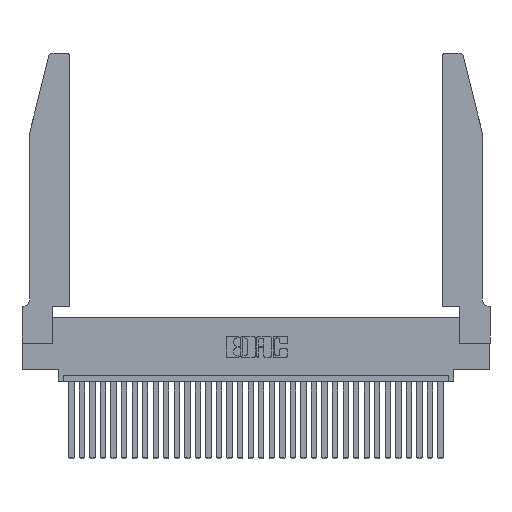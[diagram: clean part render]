
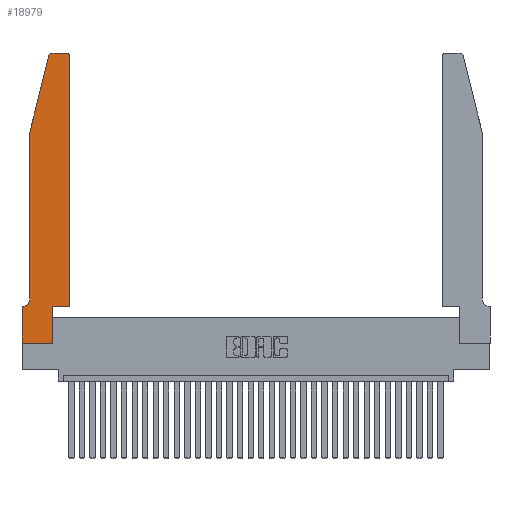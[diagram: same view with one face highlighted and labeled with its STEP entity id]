
A CAD part, top view. The second image highlights one B-rep face of the part: STEP entity #18979.
In plain terms, the highlighted planar face has unit normal (0, 0, 1).
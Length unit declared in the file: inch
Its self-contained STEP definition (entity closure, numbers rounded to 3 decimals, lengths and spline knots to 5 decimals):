
#83 = LINE ( 'NONE', #4993, #12623 ) ;
#349 = DIRECTION ( 'NONE',  ( 0., 1., 0. ) ) ;
#576 = DIRECTION ( 'NONE',  ( -1., 0., 0. ) ) ;
#654 = ORIENTED_EDGE ( 'NONE', *, *, #13467, .T. ) ;
#873 = PLANE ( 'NONE',  #4785 ) ;
#949 = ORIENTED_EDGE ( 'NONE', *, *, #26292, .T. ) ;
#970 = CARTESIAN_POINT ( 'NONE',  ( 0.2865, 0., 0.37 ) ) ;
#1658 = VECTOR ( 'NONE', #25198, 39.37008 ) ;
#1722 = VECTOR ( 'NONE', #32138, 39.37008 ) ;
#1872 = ORIENTED_EDGE ( 'NONE', *, *, #31669, .T. ) ;
#2252 = VERTEX_POINT ( 'NONE', #970 ) ;
#2437 = CARTESIAN_POINT ( 'NONE',  ( 0.2605, 2.75, 0.37 ) ) ;
#2609 = EDGE_CURVE ( 'NONE', #12792, #5001, #16962, .T. ) ;
#2851 = CARTESIAN_POINT ( 'NONE',  ( 0.4505, 0.35, 0.37 ) ) ;
#3539 = CARTESIAN_POINT ( 'NONE',  ( 0.0755, 0.42, 0.37 ) ) ;
#4785 = AXIS2_PLACEMENT_3D ( 'NONE', #5818, #31014, #18447 ) ;
#4786 = VERTEX_POINT ( 'NONE', #20227 ) ;
#4993 = CARTESIAN_POINT ( 'NONE',  ( 0.4505, 0.35, 0.37 ) ) ;
#5001 = VERTEX_POINT ( 'NONE', #8666 ) ;
#5353 = VERTEX_POINT ( 'NONE', #7013 ) ;
#5653 = CIRCLE ( 'NONE', #23288, 0.03 ) ;
#5818 = CARTESIAN_POINT ( 'NONE',  ( 0., 0.35, 0.37 ) ) ;
#6017 = DIRECTION ( 'NONE',  ( 1., 0., 0. ) ) ;
#6213 = VECTOR ( 'NONE', #12584, 39.37008 ) ;
#6500 = CARTESIAN_POINT ( 'NONE',  ( 0.25487, 2.72718, 0.37 ) ) ;
#6783 = CARTESIAN_POINT ( 'NONE',  ( 0.0755, 0.35, 0.37 ) ) ;
#7013 = CARTESIAN_POINT ( 'NONE',  ( 0., 0.35, 0.37 ) ) ;
#7657 = LINE ( 'NONE', #15133, #13528 ) ;
#7698 = EDGE_CURVE ( 'NONE', #23932, #23262, #24524, .T. ) ;
#7699 = ORIENTED_EDGE ( 'NONE', *, *, #22685, .T. ) ;
#7839 = CARTESIAN_POINT ( 'NONE',  ( 0.0055, 0.35, 0.37 ) ) ;
#7915 = CARTESIAN_POINT ( 'NONE',  ( 0.0055, 0.42, 0.37 ) ) ;
#8496 = EDGE_CURVE ( 'NONE', #15314, #18345, #83, .T. ) ;
#8666 = CARTESIAN_POINT ( 'NONE',  ( 0.284, 2.75, 0.37 ) ) ;
#9888 = AXIS2_PLACEMENT_3D ( 'NONE', #7915, #30484, #576 ) ;
#9970 = LINE ( 'NONE', #24410, #16223 ) ;
#10992 = CARTESIAN_POINT ( 'NONE',  ( 0.0755, 2., 0.37 ) ) ;
#11444 = LINE ( 'NONE', #6783, #19309 ) ;
#11681 = ORIENTED_EDGE ( 'NONE', *, *, #8496, .T. ) ;
#11913 = AXIS2_PLACEMENT_3D ( 'NONE', #13554, #18541, #6017 ) ;
#12584 = DIRECTION ( 'NONE',  ( 0., 1., 0. ) ) ;
#12623 = VECTOR ( 'NONE', #27321, 39.37008 ) ;
#12693 = EDGE_CURVE ( 'NONE', #5001, #23932, #5653, .T. ) ;
#12792 = VERTEX_POINT ( 'NONE', #27044 ) ;
#12850 = EDGE_CURVE ( 'NONE', #4786, #2252, #25303, .T. ) ;
#13062 = EDGE_LOOP ( 'NONE', ( #16958, #14139, #15153, #7699, #27635, #29638, #1872, #18734, #949, #11681, #30014, #654 ) ) ;
#13467 = EDGE_CURVE ( 'NONE', #32119, #12792, #19320, .T. ) ;
#13528 = VECTOR ( 'NONE', #349, 39.37008 ) ;
#13554 = CARTESIAN_POINT ( 'NONE',  ( 0.4205, 2.72, 0.37 ) ) ;
#14139 = ORIENTED_EDGE ( 'NONE', *, *, #12693, .T. ) ;
#14757 = CARTESIAN_POINT ( 'NONE',  ( 0.0755, 2., 0.37 ) ) ;
#15133 = CARTESIAN_POINT ( 'NONE',  ( 0.2865, 0.35, 0.37 ) ) ;
#15153 = ORIENTED_EDGE ( 'NONE', *, *, #7698, .T. ) ;
#15314 = VERTEX_POINT ( 'NONE', #26490 ) ;
#15515 = DIRECTION ( 'NONE',  ( -1., 0., 0. ) ) ;
#16223 = VECTOR ( 'NONE', #16707, 39.37008 ) ;
#16453 = VERTEX_POINT ( 'NONE', #3539 ) ;
#16707 = DIRECTION ( 'NONE',  ( 0., -1., 0. ) ) ;
#16958 = ORIENTED_EDGE ( 'NONE', *, *, #2609, .T. ) ;
#16962 = LINE ( 'NONE', #2437, #1658 ) ;
#17062 = EDGE_CURVE ( 'NONE', #28732, #5353, #11444, .T. ) ;
#17802 = VECTOR ( 'NONE', #25663, 39.37008 ) ;
#18345 = VERTEX_POINT ( 'NONE', #2851 ) ;
#18447 = DIRECTION ( 'NONE',  ( 1., 0., 0. ) ) ;
#18541 = DIRECTION ( 'NONE',  ( 0., 0., 1. ) ) ;
#18734 = ORIENTED_EDGE ( 'NONE', *, *, #12850, .T. ) ;
#18979 = ADVANCED_FACE ( 'NONE', ( #26708 ), #873, .T. ) ;
#19309 = VECTOR ( 'NONE', #15515, 39.37008 ) ;
#19320 = CIRCLE ( 'NONE', #11913, 0.03 ) ;
#20129 = EDGE_CURVE ( 'NONE', #18345, #32119, #28972, .T. ) ;
#20227 = CARTESIAN_POINT ( 'NONE',  ( 0., 0., 0.37 ) ) ;
#20309 = CARTESIAN_POINT ( 'NONE',  ( 0.4505, 0.35, 0.37 ) ) ;
#20522 = LINE ( 'NONE', #14757, #24057 ) ;
#21800 = CARTESIAN_POINT ( 'NONE',  ( 0.0755, 2., 0.37 ) ) ;
#22073 = CARTESIAN_POINT ( 'NONE',  ( 0., 0., 0.37 ) ) ;
#22685 = EDGE_CURVE ( 'NONE', #23262, #16453, #20522, .T. ) ;
#23262 = VERTEX_POINT ( 'NONE', #21800 ) ;
#23288 = AXIS2_PLACEMENT_3D ( 'NONE', #28017, #30804, #30583 ) ;
#23932 = VERTEX_POINT ( 'NONE', #6500 ) ;
#24057 = VECTOR ( 'NONE', #27346, 39.37008 ) ;
#24410 = CARTESIAN_POINT ( 'NONE',  ( 0., 0., 0.37 ) ) ;
#24524 = LINE ( 'NONE', #10992, #17802 ) ;
#25198 = DIRECTION ( 'NONE',  ( -1., 0., 0. ) ) ;
#25303 = LINE ( 'NONE', #22073, #1722 ) ;
#25390 = CARTESIAN_POINT ( 'NONE',  ( 0.4505, 2.72, 0.37 ) ) ;
#25663 = DIRECTION ( 'NONE',  ( -0.239, -0.971, 0. ) ) ;
#25785 = CIRCLE ( 'NONE', #9888, 0.07 ) ;
#26292 = EDGE_CURVE ( 'NONE', #2252, #15314, #7657, .T. ) ;
#26490 = CARTESIAN_POINT ( 'NONE',  ( 0.2865, 0.35, 0.37 ) ) ;
#26708 = FACE_OUTER_BOUND ( 'NONE', #13062, .T. ) ;
#27044 = CARTESIAN_POINT ( 'NONE',  ( 0.4205, 2.75, 0.37 ) ) ;
#27321 = DIRECTION ( 'NONE',  ( 1., 0., 0. ) ) ;
#27346 = DIRECTION ( 'NONE',  ( 0., -1., 0. ) ) ;
#27635 = ORIENTED_EDGE ( 'NONE', *, *, #31062, .T. ) ;
#28017 = CARTESIAN_POINT ( 'NONE',  ( 0.284, 2.72, 0.37 ) ) ;
#28732 = VERTEX_POINT ( 'NONE', #7839 ) ;
#28972 = LINE ( 'NONE', #20309, #6213 ) ;
#29638 = ORIENTED_EDGE ( 'NONE', *, *, #17062, .T. ) ;
#30014 = ORIENTED_EDGE ( 'NONE', *, *, #20129, .T. ) ;
#30484 = DIRECTION ( 'NONE',  ( 0., 0., -1. ) ) ;
#30583 = DIRECTION ( 'NONE',  ( 1., 0., 0. ) ) ;
#30804 = DIRECTION ( 'NONE',  ( 0., 0., 1. ) ) ;
#31014 = DIRECTION ( 'NONE',  ( 0., 0., 1. ) ) ;
#31062 = EDGE_CURVE ( 'NONE', #16453, #28732, #25785, .T. ) ;
#31669 = EDGE_CURVE ( 'NONE', #5353, #4786, #9970, .T. ) ;
#32119 = VERTEX_POINT ( 'NONE', #25390 ) ;
#32138 = DIRECTION ( 'NONE',  ( 1., 0., 0. ) ) ;
